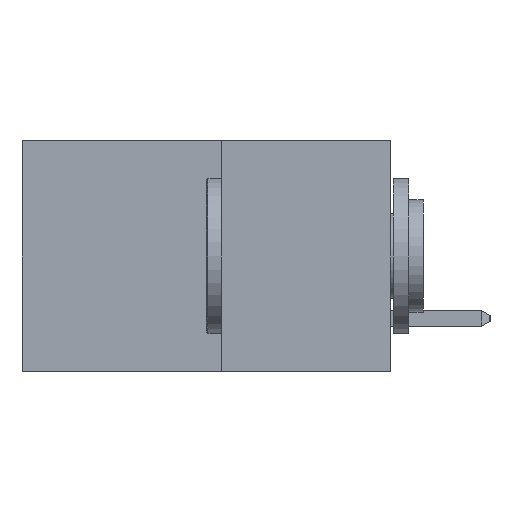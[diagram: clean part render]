
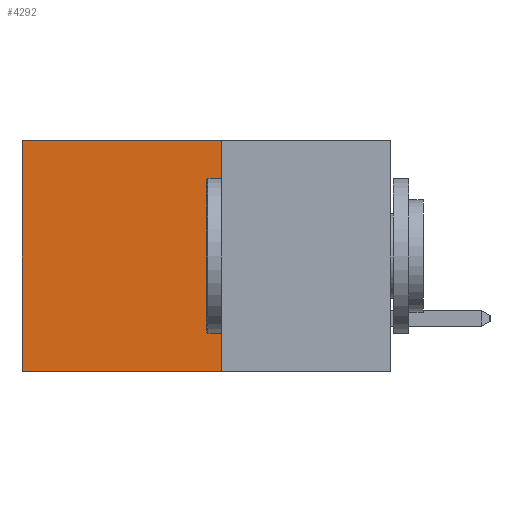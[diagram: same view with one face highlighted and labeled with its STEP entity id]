
A CAD part, left-side view. The second image highlights one B-rep face of the part: STEP entity #4292.
In plain terms, the highlighted planar face has unit normal (-1, 0, 0).
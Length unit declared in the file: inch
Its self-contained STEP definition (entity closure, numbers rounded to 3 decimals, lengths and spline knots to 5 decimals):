
#1196 = ORIENTED_EDGE ( 'NONE', *, *, #1974, .T. ) ;
#1708 = LINE ( 'NONE', #12279, #11088 ) ;
#1974 = EDGE_CURVE ( 'NONE', #5888, #5855, #6049, .T. ) ;
#2137 = DIRECTION ( 'NONE',  ( 0., 0., -1. ) ) ;
#2320 = CARTESIAN_POINT ( 'NONE',  ( 0.277, 0.59, -0.37 ) ) ;
#2771 = ORIENTED_EDGE ( 'NONE', *, *, #4064, .F. ) ;
#2887 = ORIENTED_EDGE ( 'NONE', *, *, #6863, .F. ) ;
#3137 = VERTEX_POINT ( 'NONE', #5864 ) ;
#4064 = EDGE_CURVE ( 'NONE', #3137, #6685, #11262, .T. ) ;
#4254 = EDGE_CURVE ( 'NONE', #3137, #5888, #1708, .T. ) ;
#4292 = ADVANCED_FACE ( 'NONE', ( #13406 ), #11953, .F. ) ;
#4386 = VECTOR ( 'NONE', #12739, 39.37008 ) ;
#4861 = ORIENTED_EDGE ( 'NONE', *, *, #4254, .T. ) ;
#5681 = CARTESIAN_POINT ( 'NONE',  ( 0.277, 0.59, 0. ) ) ;
#5855 = VERTEX_POINT ( 'NONE', #7049 ) ;
#5864 = CARTESIAN_POINT ( 'NONE',  ( 0.277, 0.27, 0. ) ) ;
#5888 = VERTEX_POINT ( 'NONE', #5681 ) ;
#6049 = LINE ( 'NONE', #2320, #11741 ) ;
#6685 = VERTEX_POINT ( 'NONE', #14969 ) ;
#6863 = EDGE_CURVE ( 'NONE', #6685, #5855, #10493, .T. ) ;
#7049 = CARTESIAN_POINT ( 'NONE',  ( 0.277, 0.59, -0.37 ) ) ;
#7507 = VECTOR ( 'NONE', #14057, 39.37008 ) ;
#8776 = AXIS2_PLACEMENT_3D ( 'NONE', #11971, #11938, #11922 ) ;
#9702 = EDGE_LOOP ( 'NONE', ( #1196, #2887, #2771, #4861 ) ) ;
#10493 = LINE ( 'NONE', #12775, #4386 ) ;
#11088 = VECTOR ( 'NONE', #12240, 39.37008 ) ;
#11262 = LINE ( 'NONE', #14121, #7507 ) ;
#11741 = VECTOR ( 'NONE', #2137, 39.37008 ) ;
#11922 = DIRECTION ( 'NONE',  ( 0., 0., -1. ) ) ;
#11938 = DIRECTION ( 'NONE',  ( 1., 0., 0. ) ) ;
#11953 = PLANE ( 'NONE',  #8776 ) ;
#11971 = CARTESIAN_POINT ( 'NONE',  ( 0.277, 0.27, -0.37 ) ) ;
#12240 = DIRECTION ( 'NONE',  ( 0., 1., 0. ) ) ;
#12279 = CARTESIAN_POINT ( 'NONE',  ( 0.277, 0.27, 0. ) ) ;
#12739 = DIRECTION ( 'NONE',  ( 0., 1., 0. ) ) ;
#12775 = CARTESIAN_POINT ( 'NONE',  ( 0.277, 0.27, -0.37 ) ) ;
#13406 = FACE_OUTER_BOUND ( 'NONE', #9702, .T. ) ;
#14057 = DIRECTION ( 'NONE',  ( 0., 0., -1. ) ) ;
#14121 = CARTESIAN_POINT ( 'NONE',  ( 0.277, 0.27, -0.37 ) ) ;
#14969 = CARTESIAN_POINT ( 'NONE',  ( 0.277, 0.27, -0.37 ) ) ;
